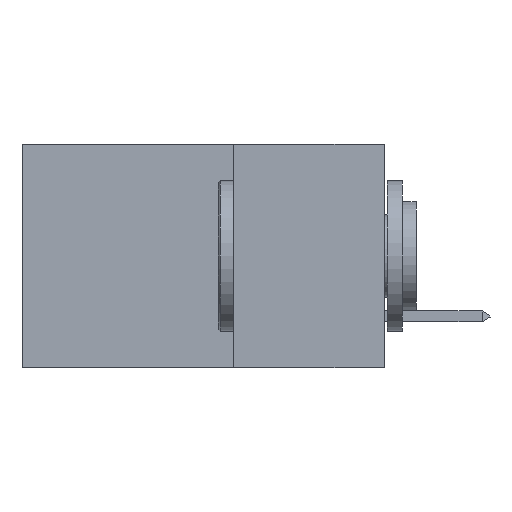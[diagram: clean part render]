
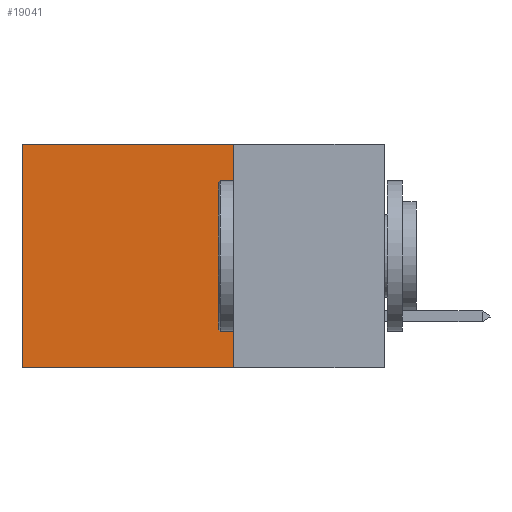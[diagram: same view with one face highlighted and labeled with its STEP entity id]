
A CAD part, left-side view. The second image highlights one B-rep face of the part: STEP entity #19041.
In plain terms, the highlighted planar face has unit normal (-1, 0, 0).
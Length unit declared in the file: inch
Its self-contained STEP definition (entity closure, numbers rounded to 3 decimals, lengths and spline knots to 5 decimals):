
#78 = LINE ( 'NONE', #4978, #16297 ) ;
#1335 = VERTEX_POINT ( 'NONE', #19053 ) ;
#2759 = DIRECTION ( 'NONE',  ( 0., 0., -1. ) ) ;
#3135 = FACE_OUTER_BOUND ( 'NONE', #16499, .T. ) ;
#4032 = DIRECTION ( 'NONE',  ( 0., 0., -1. ) ) ;
#4893 = CARTESIAN_POINT ( 'NONE',  ( 0.2875, 0.25, -0.37 ) ) ;
#4978 = CARTESIAN_POINT ( 'NONE',  ( 0.2875, 0.25, 0. ) ) ;
#5156 = DIRECTION ( 'NONE',  ( 0., 1., 0. ) ) ;
#5486 = AXIS2_PLACEMENT_3D ( 'NONE', #12298, #27237, #16387 ) ;
#6232 = ORIENTED_EDGE ( 'NONE', *, *, #22657, .T. ) ;
#6729 = VERTEX_POINT ( 'NONE', #4893 ) ;
#7403 = ORIENTED_EDGE ( 'NONE', *, *, #8304, .T. ) ;
#8056 = LINE ( 'NONE', #9316, #12328 ) ;
#8304 = EDGE_CURVE ( 'NONE', #10310, #1335, #18768, .T. ) ;
#9213 = LINE ( 'NONE', #11457, #15191 ) ;
#9316 = CARTESIAN_POINT ( 'NONE',  ( 0.2875, 0.25, -0.37 ) ) ;
#10310 = VERTEX_POINT ( 'NONE', #25589 ) ;
#11457 = CARTESIAN_POINT ( 'NONE',  ( 0.2875, 0.25, 0. ) ) ;
#12156 = CARTESIAN_POINT ( 'NONE',  ( 0.2875, 0.6, 0. ) ) ;
#12298 = CARTESIAN_POINT ( 'NONE',  ( 0.2875, 0.25, 0. ) ) ;
#12328 = VECTOR ( 'NONE', #5156, 39.37008 ) ;
#13597 = DIRECTION ( 'NONE',  ( 0., 1., 0. ) ) ;
#15191 = VECTOR ( 'NONE', #13597, 39.37008 ) ;
#15200 = ORIENTED_EDGE ( 'NONE', *, *, #25030, .F. ) ;
#16297 = VECTOR ( 'NONE', #2759, 39.37008 ) ;
#16387 = DIRECTION ( 'NONE',  ( 0., 0., -1. ) ) ;
#16499 = EDGE_LOOP ( 'NONE', ( #7403, #15200, #21137, #6232 ) ) ;
#16718 = VERTEX_POINT ( 'NONE', #18558 ) ;
#18558 = CARTESIAN_POINT ( 'NONE',  ( 0.2875, 0.25, 0. ) ) ;
#18768 = LINE ( 'NONE', #12156, #21114 ) ;
#19041 = ADVANCED_FACE ( 'NONE', ( #3135 ), #20834, .F. ) ;
#19053 = CARTESIAN_POINT ( 'NONE',  ( 0.2875, 0.6, -0.37 ) ) ;
#20834 = PLANE ( 'NONE',  #5486 ) ;
#21114 = VECTOR ( 'NONE', #4032, 39.37008 ) ;
#21137 = ORIENTED_EDGE ( 'NONE', *, *, #26536, .F. ) ;
#22657 = EDGE_CURVE ( 'NONE', #16718, #10310, #9213, .T. ) ;
#25030 = EDGE_CURVE ( 'NONE', #6729, #1335, #8056, .T. ) ;
#25589 = CARTESIAN_POINT ( 'NONE',  ( 0.2875, 0.6, 0. ) ) ;
#26536 = EDGE_CURVE ( 'NONE', #16718, #6729, #78, .T. ) ;
#27237 = DIRECTION ( 'NONE',  ( 1., 0., 0. ) ) ;
